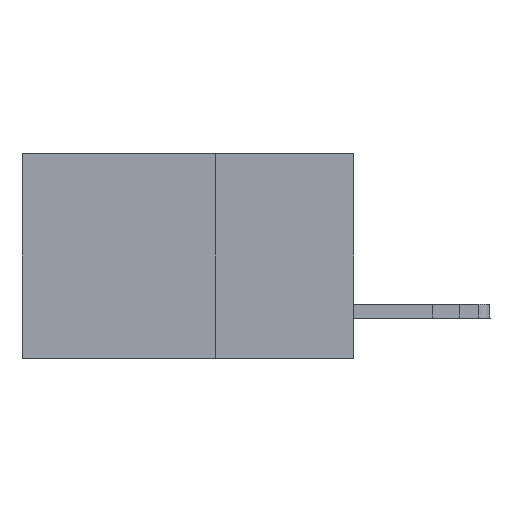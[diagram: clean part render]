
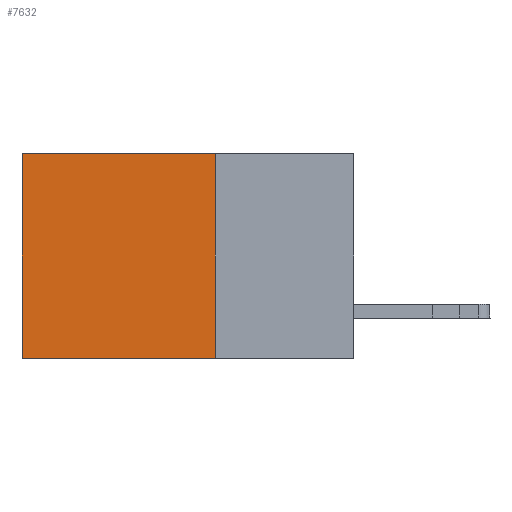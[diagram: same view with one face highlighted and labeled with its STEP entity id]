
A CAD part, left-side view. The second image highlights one B-rep face of the part: STEP entity #7632.
In plain terms, the highlighted planar face has unit normal (-1, 0, 0).
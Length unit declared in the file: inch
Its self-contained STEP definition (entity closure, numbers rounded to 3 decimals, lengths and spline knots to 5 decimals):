
#985 = DIRECTION ( 'NONE',  ( 0., 0., -1. ) ) ;
#1609 = ORIENTED_EDGE ( 'NONE', *, *, #3103, .F. ) ;
#1949 = CARTESIAN_POINT ( 'NONE',  ( 0.2875, 0.6, 0. ) ) ;
#2032 = CARTESIAN_POINT ( 'NONE',  ( 0.2875, 0.6, -0.37 ) ) ;
#2382 = CARTESIAN_POINT ( 'NONE',  ( 0.2875, 0.25, -0.37 ) ) ;
#2714 = DIRECTION ( 'NONE',  ( 0., 1., 0. ) ) ;
#2926 = VERTEX_POINT ( 'NONE', #2382 ) ;
#3103 = EDGE_CURVE ( 'NONE', #7728, #2926, #4706, .T. ) ;
#3207 = VECTOR ( 'NONE', #17733, 39.37008 ) ;
#4706 = LINE ( 'NONE', #11303, #9602 ) ;
#4932 = FACE_OUTER_BOUND ( 'NONE', #15690, .T. ) ;
#5052 = VERTEX_POINT ( 'NONE', #14414 ) ;
#5275 = EDGE_CURVE ( 'NONE', #2926, #6233, #22006, .T. ) ;
#5322 = AXIS2_PLACEMENT_3D ( 'NONE', #8194, #13839, #985 ) ;
#5658 = LINE ( 'NONE', #1949, #12432 ) ;
#6233 = VERTEX_POINT ( 'NONE', #2032 ) ;
#6482 = VECTOR ( 'NONE', #2714, 39.37008 ) ;
#7632 = ADVANCED_FACE ( 'NONE', ( #4932 ), #15345, .F. ) ;
#7728 = VERTEX_POINT ( 'NONE', #8302 ) ;
#8194 = CARTESIAN_POINT ( 'NONE',  ( 0.2875, 0.25, 0. ) ) ;
#8302 = CARTESIAN_POINT ( 'NONE',  ( 0.2875, 0.25, 0. ) ) ;
#9602 = VECTOR ( 'NONE', #11749, 39.37008 ) ;
#11303 = CARTESIAN_POINT ( 'NONE',  ( 0.2875, 0.25, 0. ) ) ;
#11749 = DIRECTION ( 'NONE',  ( 0., 0., -1. ) ) ;
#11915 = EDGE_CURVE ( 'NONE', #7728, #5052, #21511, .T. ) ;
#12432 = VECTOR ( 'NONE', #12608, 39.37008 ) ;
#12608 = DIRECTION ( 'NONE',  ( 0., 0., -1. ) ) ;
#13839 = DIRECTION ( 'NONE',  ( 1., 0., 0. ) ) ;
#14049 = EDGE_CURVE ( 'NONE', #5052, #6233, #5658, .T. ) ;
#14414 = CARTESIAN_POINT ( 'NONE',  ( 0.2875, 0.6, 0. ) ) ;
#15345 = PLANE ( 'NONE',  #5322 ) ;
#15690 = EDGE_LOOP ( 'NONE', ( #19789, #18995, #1609, #16969 ) ) ;
#16969 = ORIENTED_EDGE ( 'NONE', *, *, #11915, .T. ) ;
#17733 = DIRECTION ( 'NONE',  ( 0., 1., 0. ) ) ;
#18995 = ORIENTED_EDGE ( 'NONE', *, *, #5275, .F. ) ;
#19780 = CARTESIAN_POINT ( 'NONE',  ( 0.2875, 0.25, 0. ) ) ;
#19789 = ORIENTED_EDGE ( 'NONE', *, *, #14049, .T. ) ;
#20723 = CARTESIAN_POINT ( 'NONE',  ( 0.2875, 0.25, -0.37 ) ) ;
#21511 = LINE ( 'NONE', #19780, #3207 ) ;
#22006 = LINE ( 'NONE', #20723, #6482 ) ;
